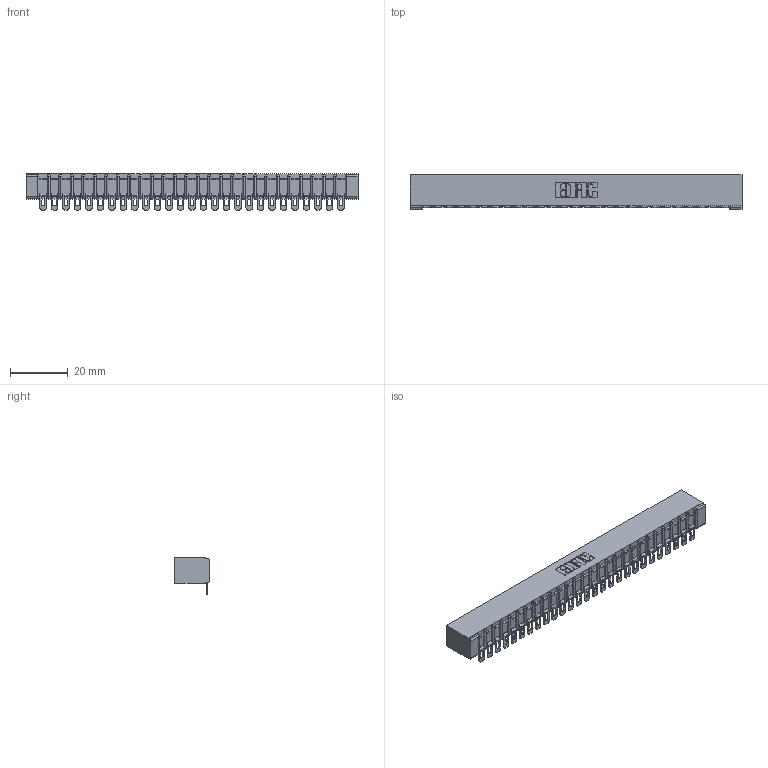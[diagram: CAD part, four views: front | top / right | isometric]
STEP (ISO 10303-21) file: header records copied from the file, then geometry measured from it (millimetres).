
FILE_DESCRIPTION (( 'STEP AP203' ), '1' );
FILE_NAME ('307-027-454-101.STEP', '2020-09-28T05:44:46', ( '' ), ( '' ), 'SwSTEP 2.0', 'SolidWorks 2020', '' );
FILE_SCHEMA (( 'CONFIG_CONTROL_DESIGN' ));
Length unit declared in the file: inch
Products named in the file (3): 307 Part_No Mounting Lugs; 307-027-454-101; 307-290-002_554
Assembly tree (28 placements, depth 2):
  307-027-454-101
    307 Part_No Mounting Lugs
    307-290-002_554  x27
Bounding box: 114.86 x 12.01 x 12.52 mm (x, y, z)
Volume: 7837.4 mm3; surface area: 15151.3 mm2
Topology: 28 solids, 28 shells, 2325 faces, 7130 edges, 4676 vertices
Faces by surface type: plane 1308, cylinder 961, sphere 56
Entity records: 25683 total; most frequent: CARTESIAN_POINT 4330, ORIENTED_EDGE 4320, DIRECTION 4218, EDGE_CURVE 2160, LINE 1642, VECTOR 1642, VERTEX_POINT 1400, AXIS2_PLACEMENT_3D 1288
